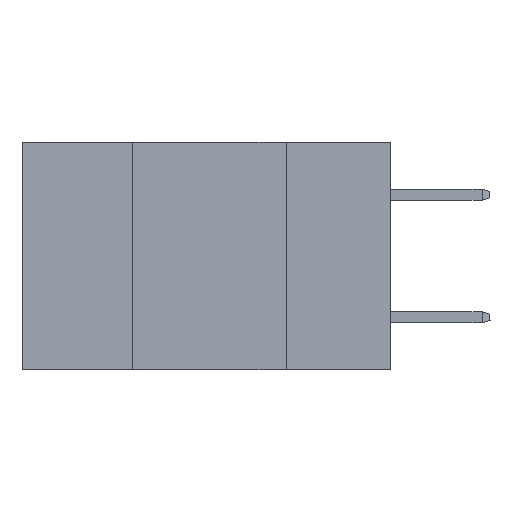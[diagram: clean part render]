
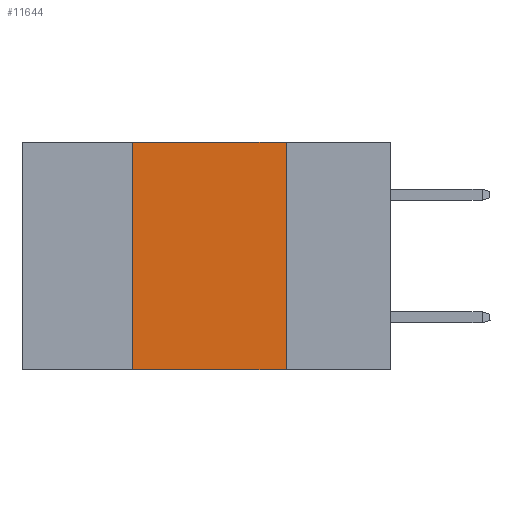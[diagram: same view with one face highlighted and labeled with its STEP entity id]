
A CAD part, left-side view. The second image highlights one B-rep face of the part: STEP entity #11644.
In plain terms, the highlighted planar face has unit normal (-1, 0, 0).
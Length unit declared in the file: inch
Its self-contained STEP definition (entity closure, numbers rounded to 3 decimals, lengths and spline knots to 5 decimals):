
#273 = DIRECTION ( 'NONE',  ( 0., -1., 0. ) ) ;
#546 = ORIENTED_EDGE ( 'NONE', *, *, #2029, .F. ) ;
#1327 = LINE ( 'NONE', #2789, #14816 ) ;
#1667 = DIRECTION ( 'NONE',  ( 0., -1., 0. ) ) ;
#2029 = EDGE_CURVE ( 'NONE', #8774, #16343, #1327, .T. ) ;
#2696 = VERTEX_POINT ( 'NONE', #12147 ) ;
#2789 = CARTESIAN_POINT ( 'NONE',  ( 0., 0.17, 0. ) ) ;
#3014 = CARTESIAN_POINT ( 'NONE',  ( 0., 0.17, 0. ) ) ;
#3064 = CARTESIAN_POINT ( 'NONE',  ( 0., 0.6, 0. ) ) ;
#3086 = CARTESIAN_POINT ( 'NONE',  ( 0., 0.42, -0.37 ) ) ;
#3186 = DIRECTION ( 'NONE',  ( 0., 0., 1. ) ) ;
#3403 = VECTOR ( 'NONE', #1667, 39.37008 ) ;
#4275 = AXIS2_PLACEMENT_3D ( 'NONE', #3064, #4397, #14821 ) ;
#4392 = CARTESIAN_POINT ( 'NONE',  ( 0., 0.6, -0.37 ) ) ;
#4397 = DIRECTION ( 'NONE',  ( 1., 0., 0. ) ) ;
#4496 = EDGE_LOOP ( 'NONE', ( #546, #13405, #8569, #6410 ) ) ;
#4540 = EDGE_CURVE ( 'NONE', #2696, #8774, #6260, .T. ) ;
#5146 = CARTESIAN_POINT ( 'NONE',  ( 0., 0.6, 0. ) ) ;
#6260 = LINE ( 'NONE', #5146, #3403 ) ;
#6410 = ORIENTED_EDGE ( 'NONE', *, *, #10945, .T. ) ;
#6727 = VECTOR ( 'NONE', #273, 39.37008 ) ;
#6740 = DIRECTION ( 'NONE',  ( 0., 0., -1. ) ) ;
#7134 = PLANE ( 'NONE',  #4275 ) ;
#7155 = LINE ( 'NONE', #4392, #6727 ) ;
#7644 = VECTOR ( 'NONE', #3186, 39.37008 ) ;
#8433 = EDGE_CURVE ( 'NONE', #11952, #2696, #12549, .T. ) ;
#8569 = ORIENTED_EDGE ( 'NONE', *, *, #8433, .F. ) ;
#8774 = VERTEX_POINT ( 'NONE', #3014 ) ;
#10945 = EDGE_CURVE ( 'NONE', #11952, #16343, #7155, .T. ) ;
#10994 = CARTESIAN_POINT ( 'NONE',  ( 0., 0.42, 0. ) ) ;
#11644 = ADVANCED_FACE ( 'NONE', ( #12403 ), #7134, .F. ) ;
#11952 = VERTEX_POINT ( 'NONE', #3086 ) ;
#12133 = CARTESIAN_POINT ( 'NONE',  ( 0., 0.17, -0.37 ) ) ;
#12147 = CARTESIAN_POINT ( 'NONE',  ( 0., 0.42, 0. ) ) ;
#12403 = FACE_OUTER_BOUND ( 'NONE', #4496, .T. ) ;
#12549 = LINE ( 'NONE', #10994, #7644 ) ;
#13405 = ORIENTED_EDGE ( 'NONE', *, *, #4540, .F. ) ;
#14816 = VECTOR ( 'NONE', #6740, 39.37008 ) ;
#14821 = DIRECTION ( 'NONE',  ( 0., 0., -1. ) ) ;
#16343 = VERTEX_POINT ( 'NONE', #12133 ) ;
